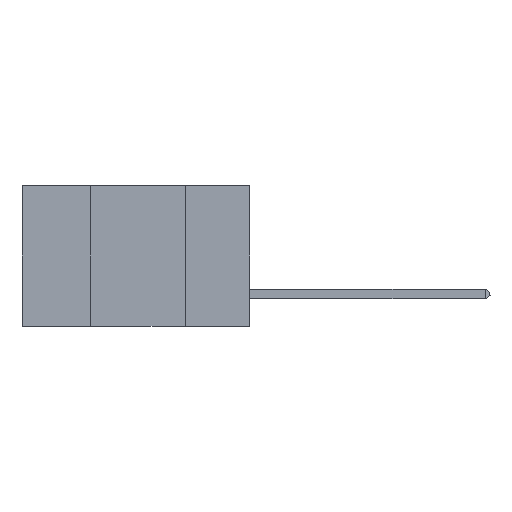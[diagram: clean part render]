
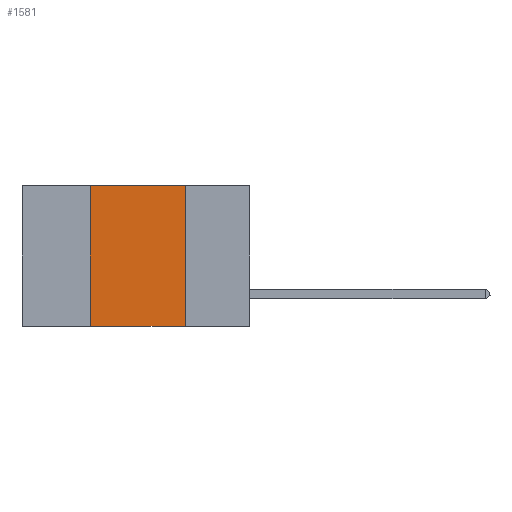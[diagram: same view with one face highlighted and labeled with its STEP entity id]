
A CAD part, left-side view. The second image highlights one B-rep face of the part: STEP entity #1581.
In plain terms, the highlighted planar face has unit normal (-1, 0, 0).
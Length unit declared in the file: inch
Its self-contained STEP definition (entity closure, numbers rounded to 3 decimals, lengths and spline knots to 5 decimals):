
#390 = VECTOR ( 'NONE', #9634, 39.37008 ) ;
#806 = PLANE ( 'NONE',  #7029 ) ;
#1581 = ADVANCED_FACE ( 'NONE', ( #5372 ), #806, .F. ) ;
#2360 = VERTEX_POINT ( 'NONE', #5661 ) ;
#2561 = VERTEX_POINT ( 'NONE', #10136 ) ;
#2895 = EDGE_CURVE ( 'NONE', #2360, #9258, #3542, .T. ) ;
#2904 = DIRECTION ( 'NONE',  ( 0., 0., 1. ) ) ;
#3116 = CARTESIAN_POINT ( 'NONE',  ( 0., 0.42, -0.37 ) ) ;
#3542 = LINE ( 'NONE', #8417, #9850 ) ;
#4169 = ORIENTED_EDGE ( 'NONE', *, *, #7739, .F. ) ;
#4191 = EDGE_CURVE ( 'NONE', #8565, #9258, #9044, .T. ) ;
#4817 = DIRECTION ( 'NONE',  ( 0., 0., -1. ) ) ;
#4865 = DIRECTION ( 'NONE',  ( 0., -1., 0. ) ) ;
#4983 = DIRECTION ( 'NONE',  ( 1., 0., 0. ) ) ;
#5372 = FACE_OUTER_BOUND ( 'NONE', #5771, .T. ) ;
#5396 = ORIENTED_EDGE ( 'NONE', *, *, #4191, .T. ) ;
#5496 = CARTESIAN_POINT ( 'NONE',  ( 0., 0.6, 0. ) ) ;
#5661 = CARTESIAN_POINT ( 'NONE',  ( 0., 0.17, 0. ) ) ;
#5771 = EDGE_LOOP ( 'NONE', ( #7430, #4169, #10762, #5396 ) ) ;
#6555 = EDGE_CURVE ( 'NONE', #8565, #2561, #6841, .T. ) ;
#6612 = CARTESIAN_POINT ( 'NONE',  ( 0., 0.6, 0. ) ) ;
#6841 = LINE ( 'NONE', #7015, #10715 ) ;
#7015 = CARTESIAN_POINT ( 'NONE',  ( 0., 0.42, 0. ) ) ;
#7029 = AXIS2_PLACEMENT_3D ( 'NONE', #6612, #4983, #7477 ) ;
#7430 = ORIENTED_EDGE ( 'NONE', *, *, #2895, .F. ) ;
#7477 = DIRECTION ( 'NONE',  ( 0., 0., -1. ) ) ;
#7739 = EDGE_CURVE ( 'NONE', #2561, #2360, #9125, .T. ) ;
#8230 = CARTESIAN_POINT ( 'NONE',  ( 0., 0.17, -0.37 ) ) ;
#8417 = CARTESIAN_POINT ( 'NONE',  ( 0., 0.17, 0. ) ) ;
#8565 = VERTEX_POINT ( 'NONE', #3116 ) ;
#8999 = CARTESIAN_POINT ( 'NONE',  ( 0., 0.6, -0.37 ) ) ;
#9044 = LINE ( 'NONE', #8999, #9300 ) ;
#9125 = LINE ( 'NONE', #5496, #390 ) ;
#9258 = VERTEX_POINT ( 'NONE', #8230 ) ;
#9300 = VECTOR ( 'NONE', #4865, 39.37008 ) ;
#9634 = DIRECTION ( 'NONE',  ( 0., -1., 0. ) ) ;
#9850 = VECTOR ( 'NONE', #4817, 39.37008 ) ;
#10136 = CARTESIAN_POINT ( 'NONE',  ( 0., 0.42, 0. ) ) ;
#10715 = VECTOR ( 'NONE', #2904, 39.37008 ) ;
#10762 = ORIENTED_EDGE ( 'NONE', *, *, #6555, .F. ) ;
